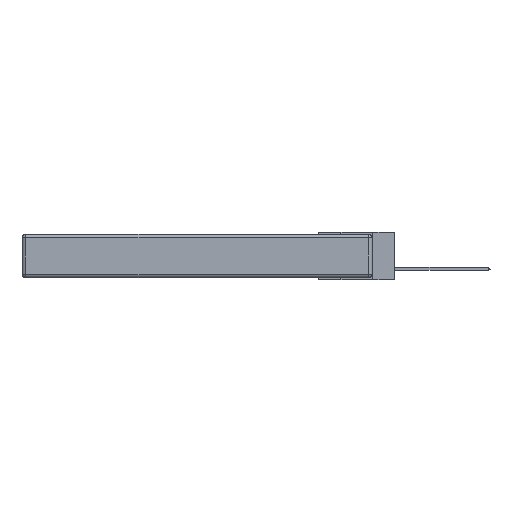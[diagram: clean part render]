
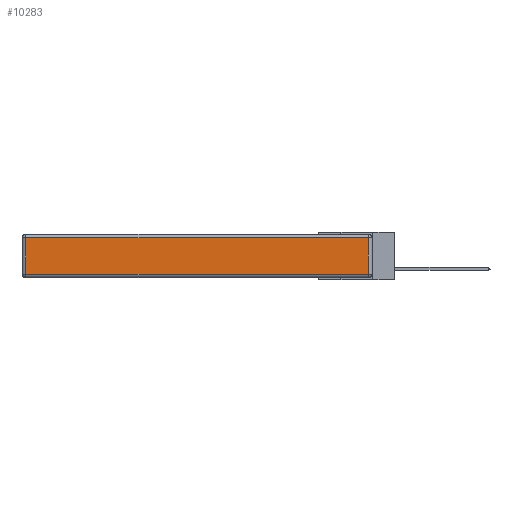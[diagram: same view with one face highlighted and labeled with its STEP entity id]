
A CAD part, left-side view. The second image highlights one B-rep face of the part: STEP entity #10283.
In plain terms, the highlighted planar face has unit normal (-1, 0, 0).
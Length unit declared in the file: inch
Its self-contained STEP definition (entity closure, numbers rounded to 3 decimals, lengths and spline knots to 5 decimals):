
#1577 = CARTESIAN_POINT ( 'NONE',  ( 0., 0., -0.343 ) ) ;
#2295 = CARTESIAN_POINT ( 'NONE',  ( 0., 2.72, -0.343 ) ) ;
#3219 = VECTOR ( 'NONE', #20421, 39.37008 ) ;
#3687 = CARTESIAN_POINT ( 'NONE',  ( 0., 0.03, -0.343 ) ) ;
#3945 = VECTOR ( 'NONE', #4557, 39.37008 ) ;
#4557 = DIRECTION ( 'NONE',  ( 0., 0., -1. ) ) ;
#5049 = VERTEX_POINT ( 'NONE', #6576 ) ;
#6223 = DIRECTION ( 'NONE',  ( 0., 1., 0. ) ) ;
#6576 = CARTESIAN_POINT ( 'NONE',  ( 0., 0.03, -0.03 ) ) ;
#6663 = LINE ( 'NONE', #13215, #17574 ) ;
#6715 = DIRECTION ( 'NONE',  ( 0., 0., 1. ) ) ;
#7201 = CARTESIAN_POINT ( 'NONE',  ( 0., 2.72, -0.313 ) ) ;
#8334 = ORIENTED_EDGE ( 'NONE', *, *, #13371, .T. ) ;
#9123 = ORIENTED_EDGE ( 'NONE', *, *, #25253, .T. ) ;
#10283 = ADVANCED_FACE ( 'NONE', ( #20136 ), #17253, .T. ) ;
#10339 = LINE ( 'NONE', #2295, #3945 ) ;
#10407 = EDGE_LOOP ( 'NONE', ( #9123, #8334, #18035, #19095 ) ) ;
#12382 = LINE ( 'NONE', #22312, #3219 ) ;
#12701 = DIRECTION ( 'NONE',  ( -1., 0., 0. ) ) ;
#13215 = CARTESIAN_POINT ( 'NONE',  ( 0., 2.75, -0.03 ) ) ;
#13371 = EDGE_CURVE ( 'NONE', #13912, #5049, #26610, .T. ) ;
#13912 = VERTEX_POINT ( 'NONE', #27833 ) ;
#16482 = EDGE_CURVE ( 'NONE', #5049, #17994, #6663, .T. ) ;
#17253 = PLANE ( 'NONE',  #24457 ) ;
#17574 = VECTOR ( 'NONE', #6223, 39.37008 ) ;
#17994 = VERTEX_POINT ( 'NONE', #25498 ) ;
#18035 = ORIENTED_EDGE ( 'NONE', *, *, #16482, .T. ) ;
#19095 = ORIENTED_EDGE ( 'NONE', *, *, #23527, .T. ) ;
#20136 = FACE_OUTER_BOUND ( 'NONE', #10407, .T. ) ;
#20421 = DIRECTION ( 'NONE',  ( 0., -1., 0. ) ) ;
#20608 = VECTOR ( 'NONE', #28352, 39.37008 ) ;
#22312 = CARTESIAN_POINT ( 'NONE',  ( 0., 0., -0.313 ) ) ;
#23527 = EDGE_CURVE ( 'NONE', #17994, #26532, #10339, .T. ) ;
#24457 = AXIS2_PLACEMENT_3D ( 'NONE', #1577, #12701, #6715 ) ;
#25253 = EDGE_CURVE ( 'NONE', #26532, #13912, #12382, .T. ) ;
#25498 = CARTESIAN_POINT ( 'NONE',  ( 0., 2.72, -0.03 ) ) ;
#26532 = VERTEX_POINT ( 'NONE', #7201 ) ;
#26610 = LINE ( 'NONE', #3687, #20608 ) ;
#27833 = CARTESIAN_POINT ( 'NONE',  ( 0., 0.03, -0.313 ) ) ;
#28352 = DIRECTION ( 'NONE',  ( 0., 0., 1. ) ) ;
